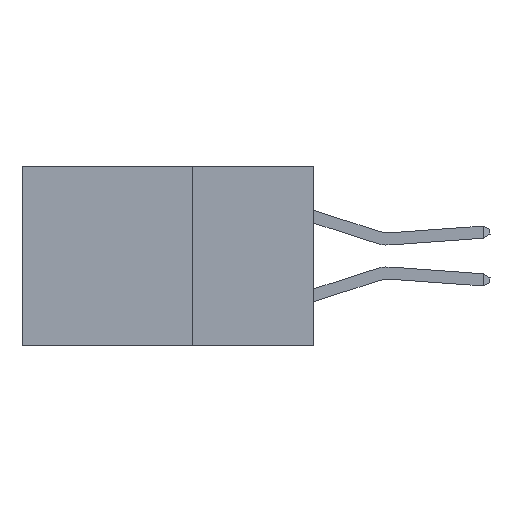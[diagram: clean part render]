
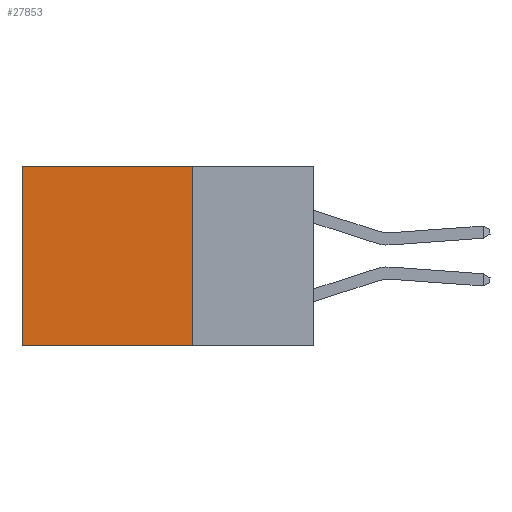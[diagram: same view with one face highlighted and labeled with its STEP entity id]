
A CAD part, left-side view. The second image highlights one B-rep face of the part: STEP entity #27853.
In plain terms, the highlighted planar face has unit normal (-1, 0, 0).
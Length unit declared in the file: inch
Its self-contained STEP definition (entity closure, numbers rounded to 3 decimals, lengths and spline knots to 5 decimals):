
#2023 = CARTESIAN_POINT ( 'NONE',  ( 0.2875, 0.25, 0. ) ) ;
#3878 = CARTESIAN_POINT ( 'NONE',  ( 0.2875, 0.25, -0.37 ) ) ;
#3935 = DIRECTION ( 'NONE',  ( 0., 0., -1. ) ) ;
#4979 = ORIENTED_EDGE ( 'NONE', *, *, #24322, .F. ) ;
#5003 = EDGE_CURVE ( 'NONE', #6004, #28940, #13024, .T. ) ;
#6004 = VERTEX_POINT ( 'NONE', #26908 ) ;
#6333 = VECTOR ( 'NONE', #11697, 39.37008 ) ;
#7317 = CARTESIAN_POINT ( 'NONE',  ( 0.2875, 0.25, 0. ) ) ;
#7798 = ORIENTED_EDGE ( 'NONE', *, *, #15916, .F. ) ;
#8461 = PLANE ( 'NONE',  #22116 ) ;
#9663 = DIRECTION ( 'NONE',  ( 0., 0., -1. ) ) ;
#10052 = EDGE_CURVE ( 'NONE', #18094, #6004, #31894, .T. ) ;
#10442 = EDGE_LOOP ( 'NONE', ( #27658, #4979, #7798, #30044 ) ) ;
#10650 = LINE ( 'NONE', #11807, #6333 ) ;
#11697 = DIRECTION ( 'NONE',  ( 0., 1., 0. ) ) ;
#11807 = CARTESIAN_POINT ( 'NONE',  ( 0.2875, 0.25, -0.37 ) ) ;
#11842 = LINE ( 'NONE', #2023, #22028 ) ;
#13024 = LINE ( 'NONE', #14018, #20846 ) ;
#14018 = CARTESIAN_POINT ( 'NONE',  ( 0.2875, 0.6, 0. ) ) ;
#14126 = FACE_OUTER_BOUND ( 'NONE', #10442, .T. ) ;
#15916 = EDGE_CURVE ( 'NONE', #18094, #18436, #11842, .T. ) ;
#18094 = VERTEX_POINT ( 'NONE', #19689 ) ;
#18436 = VERTEX_POINT ( 'NONE', #3878 ) ;
#19689 = CARTESIAN_POINT ( 'NONE',  ( 0.2875, 0.25, 0. ) ) ;
#20843 = CARTESIAN_POINT ( 'NONE',  ( 0.2875, 0.6, -0.37 ) ) ;
#20846 = VECTOR ( 'NONE', #3935, 39.37008 ) ;
#22028 = VECTOR ( 'NONE', #9663, 39.37008 ) ;
#22116 = AXIS2_PLACEMENT_3D ( 'NONE', #31118, #23683, #31231 ) ;
#23683 = DIRECTION ( 'NONE',  ( 1., 0., 0. ) ) ;
#24322 = EDGE_CURVE ( 'NONE', #18436, #28940, #10650, .T. ) ;
#24736 = DIRECTION ( 'NONE',  ( 0., 1., 0. ) ) ;
#25203 = VECTOR ( 'NONE', #24736, 39.37008 ) ;
#26908 = CARTESIAN_POINT ( 'NONE',  ( 0.2875, 0.6, 0. ) ) ;
#27658 = ORIENTED_EDGE ( 'NONE', *, *, #5003, .T. ) ;
#27853 = ADVANCED_FACE ( 'NONE', ( #14126 ), #8461, .F. ) ;
#28940 = VERTEX_POINT ( 'NONE', #20843 ) ;
#30044 = ORIENTED_EDGE ( 'NONE', *, *, #10052, .T. ) ;
#31118 = CARTESIAN_POINT ( 'NONE',  ( 0.2875, 0.25, 0. ) ) ;
#31231 = DIRECTION ( 'NONE',  ( 0., 0., -1. ) ) ;
#31894 = LINE ( 'NONE', #7317, #25203 ) ;
